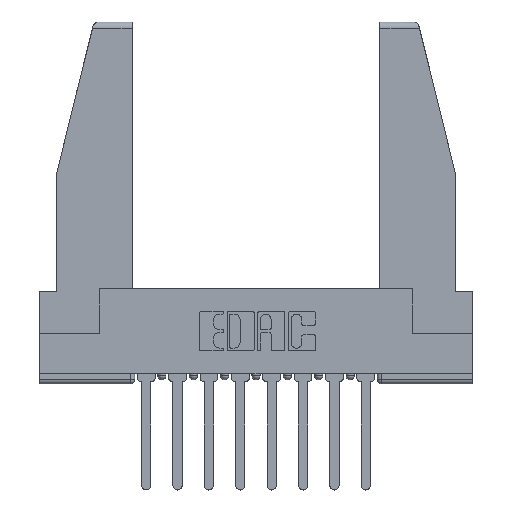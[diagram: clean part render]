
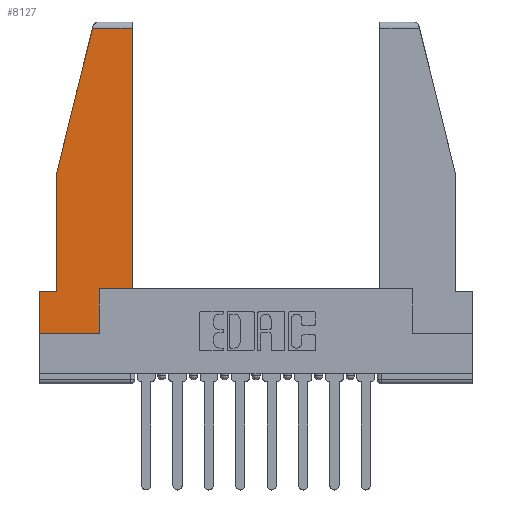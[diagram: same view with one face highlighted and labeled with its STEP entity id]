
A CAD part, top view. The second image highlights one B-rep face of the part: STEP entity #8127.
In plain terms, the highlighted planar face has unit normal (0, 0, 1).
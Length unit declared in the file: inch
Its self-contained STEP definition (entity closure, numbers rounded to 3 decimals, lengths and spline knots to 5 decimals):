
#498 = CARTESIAN_POINT ( 'NONE',  ( 0.297, 0., 0. ) ) ;
#772 = VERTEX_POINT ( 'NONE', #11732 ) ;
#997 = DIRECTION ( 'NONE',  ( 1., 0., 0. ) ) ;
#1185 = DIRECTION ( 'NONE',  ( 0., -1., 0. ) ) ;
#1237 = EDGE_CURVE ( 'NONE', #3245, #7145, #5350, .T. ) ;
#1485 = EDGE_CURVE ( 'NONE', #8675, #1826, #3813, .T. ) ;
#1542 = CARTESIAN_POINT ( 'NONE',  ( 0.461, 1.52, 0. ) ) ;
#1826 = VERTEX_POINT ( 'NONE', #1542 ) ;
#1913 = LINE ( 'NONE', #9373, #5874 ) ;
#2097 = CARTESIAN_POINT ( 'NONE',  ( 0., 0., 0. ) ) ;
#2209 = CARTESIAN_POINT ( 'NONE',  ( 0., 0., 0. ) ) ;
#2528 = LINE ( 'NONE', #6902, #5482 ) ;
#2532 = CARTESIAN_POINT ( 'NONE',  ( 0.461, 0.223, 0. ) ) ;
#3189 = ORIENTED_EDGE ( 'NONE', *, *, #8043, .T. ) ;
#3194 = VECTOR ( 'NONE', #8360, 39.37008 ) ;
#3207 = CARTESIAN_POINT ( 'NONE',  ( 0.086, 0.8, 0. ) ) ;
#3245 = VERTEX_POINT ( 'NONE', #3800 ) ;
#3764 = VECTOR ( 'NONE', #997, 39.37008 ) ;
#3800 = CARTESIAN_POINT ( 'NONE',  ( 0.2636, 1.52, 0. ) ) ;
#3813 = LINE ( 'NONE', #5252, #12677 ) ;
#4104 = CARTESIAN_POINT ( 'NONE',  ( 0.086, 0.21, 0. ) ) ;
#4688 = EDGE_CURVE ( 'NONE', #7554, #772, #12300, .T. ) ;
#5252 = CARTESIAN_POINT ( 'NONE',  ( 0.461, 0.223, 0. ) ) ;
#5350 = LINE ( 'NONE', #12888, #9686 ) ;
#5397 = ORIENTED_EDGE ( 'NONE', *, *, #1485, .T. ) ;
#5409 = PLANE ( 'NONE',  #8080 ) ;
#5482 = VECTOR ( 'NONE', #6761, 39.37008 ) ;
#5581 = EDGE_LOOP ( 'NONE', ( #5397, #3189, #8001, #9640, #6104, #6264, #7956, #6992, #10102 ) ) ;
#5718 = EDGE_CURVE ( 'NONE', #7468, #8675, #2528, .T. ) ;
#5874 = VECTOR ( 'NONE', #12319, 39.37008 ) ;
#5910 = CARTESIAN_POINT ( 'NONE',  ( 0.297, 0.223, 0. ) ) ;
#6104 = ORIENTED_EDGE ( 'NONE', *, *, #4688, .T. ) ;
#6264 = ORIENTED_EDGE ( 'NONE', *, *, #7135, .T. ) ;
#6761 = DIRECTION ( 'NONE',  ( 1., 0., 0. ) ) ;
#6902 = CARTESIAN_POINT ( 'NONE',  ( 0.297, 0.223, 0. ) ) ;
#6917 = CARTESIAN_POINT ( 'NONE',  ( 0., 0.21, 0. ) ) ;
#6992 = ORIENTED_EDGE ( 'NONE', *, *, #7985, .T. ) ;
#7033 = VECTOR ( 'NONE', #1185, 39.37008 ) ;
#7044 = VECTOR ( 'NONE', #13431, 39.37008 ) ;
#7135 = EDGE_CURVE ( 'NONE', #772, #8449, #9469, .T. ) ;
#7145 = VERTEX_POINT ( 'NONE', #7949 ) ;
#7415 = DIRECTION ( 'NONE',  ( 0., 0., 1. ) ) ;
#7468 = VERTEX_POINT ( 'NONE', #5910 ) ;
#7489 = FACE_OUTER_BOUND ( 'NONE', #5581, .T. ) ;
#7554 = VERTEX_POINT ( 'NONE', #4104 ) ;
#7949 = CARTESIAN_POINT ( 'NONE',  ( 0.086, 0.8, 0. ) ) ;
#7956 = ORIENTED_EDGE ( 'NONE', *, *, #11389, .T. ) ;
#7985 = EDGE_CURVE ( 'NONE', #8301, #7468, #11210, .T. ) ;
#8001 = ORIENTED_EDGE ( 'NONE', *, *, #1237, .T. ) ;
#8043 = EDGE_CURVE ( 'NONE', #1826, #3245, #1913, .T. ) ;
#8080 = AXIS2_PLACEMENT_3D ( 'NONE', #2209, #7415, #9712 ) ;
#8127 = ADVANCED_FACE ( 'NONE', ( #7489 ), #5409, .T. ) ;
#8301 = VERTEX_POINT ( 'NONE', #498 ) ;
#8325 = CARTESIAN_POINT ( 'NONE',  ( 0.297, 0., 0. ) ) ;
#8360 = DIRECTION ( 'NONE',  ( 0., -1., 0. ) ) ;
#8449 = VERTEX_POINT ( 'NONE', #11124 ) ;
#8482 = LINE ( 'NONE', #3207, #7033 ) ;
#8499 = LINE ( 'NONE', #2097, #3764 ) ;
#8675 = VERTEX_POINT ( 'NONE', #2532 ) ;
#8747 = DIRECTION ( 'NONE',  ( -0.239, -0.971, 0. ) ) ;
#9094 = DIRECTION ( 'NONE',  ( 0., 1., 0. ) ) ;
#9373 = CARTESIAN_POINT ( 'NONE',  ( 0., 1.52, 0. ) ) ;
#9469 = LINE ( 'NONE', #6917, #3194 ) ;
#9640 = ORIENTED_EDGE ( 'NONE', *, *, #13154, .T. ) ;
#9686 = VECTOR ( 'NONE', #8747, 39.37008 ) ;
#9712 = DIRECTION ( 'NONE',  ( 1., 0., 0. ) ) ;
#10102 = ORIENTED_EDGE ( 'NONE', *, *, #5718, .T. ) ;
#11124 = CARTESIAN_POINT ( 'NONE',  ( 0., 0., 0. ) ) ;
#11205 = DIRECTION ( 'NONE',  ( 0., 1., 0. ) ) ;
#11210 = LINE ( 'NONE', #8325, #11387 ) ;
#11387 = VECTOR ( 'NONE', #9094, 39.37008 ) ;
#11389 = EDGE_CURVE ( 'NONE', #8449, #8301, #8499, .T. ) ;
#11553 = CARTESIAN_POINT ( 'NONE',  ( 0., 0.21, 0. ) ) ;
#11732 = CARTESIAN_POINT ( 'NONE',  ( 0., 0.21, 0. ) ) ;
#12300 = LINE ( 'NONE', #11553, #7044 ) ;
#12319 = DIRECTION ( 'NONE',  ( -1., 0., 0. ) ) ;
#12677 = VECTOR ( 'NONE', #11205, 39.37008 ) ;
#12888 = CARTESIAN_POINT ( 'NONE',  ( 0.271, 1.55, 0. ) ) ;
#13154 = EDGE_CURVE ( 'NONE', #7145, #7554, #8482, .T. ) ;
#13431 = DIRECTION ( 'NONE',  ( -1., 0., 0. ) ) ;
